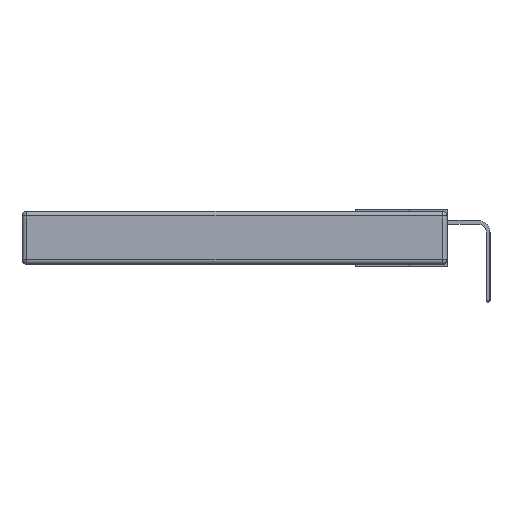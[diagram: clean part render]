
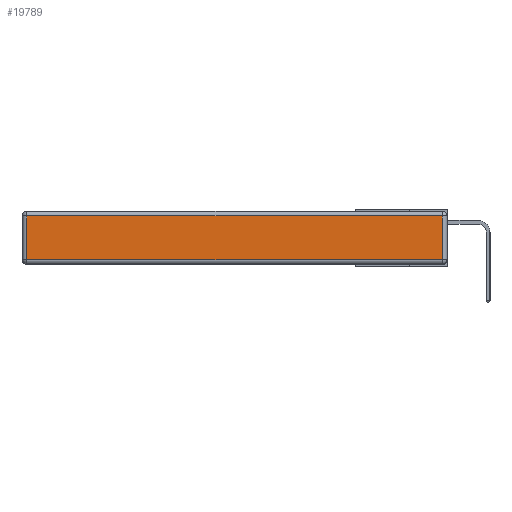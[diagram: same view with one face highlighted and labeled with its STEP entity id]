
A CAD part, left-side view. The second image highlights one B-rep face of the part: STEP entity #19789.
In plain terms, the highlighted planar face has unit normal (-1, 0, 0).
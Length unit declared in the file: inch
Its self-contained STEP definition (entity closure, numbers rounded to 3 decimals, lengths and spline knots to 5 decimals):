
#1203 = EDGE_CURVE ( 'NONE', #19280, #5224, #28338, .T. ) ;
#1354 = ORIENTED_EDGE ( 'NONE', *, *, #30653, .T. ) ;
#1513 = CARTESIAN_POINT ( 'NONE',  ( 0., 2.72, -0.343 ) ) ;
#2247 = CARTESIAN_POINT ( 'NONE',  ( 0., 2.72, -0.03 ) ) ;
#2945 = EDGE_CURVE ( 'NONE', #28315, #19280, #23787, .T. ) ;
#4897 = CARTESIAN_POINT ( 'NONE',  ( 0., 0., -0.343 ) ) ;
#5224 = VERTEX_POINT ( 'NONE', #20576 ) ;
#5275 = VECTOR ( 'NONE', #21024, 39.37008 ) ;
#6289 = EDGE_CURVE ( 'NONE', #5224, #21996, #17674, .T. ) ;
#6889 = LINE ( 'NONE', #13466, #11385 ) ;
#7324 = VECTOR ( 'NONE', #28319, 39.37008 ) ;
#9633 = AXIS2_PLACEMENT_3D ( 'NONE', #4897, #23283, #20837 ) ;
#9774 = FACE_OUTER_BOUND ( 'NONE', #18706, .T. ) ;
#11385 = VECTOR ( 'NONE', #18555, 39.37008 ) ;
#13466 = CARTESIAN_POINT ( 'NONE',  ( 0., 0.03, -0.343 ) ) ;
#15221 = ORIENTED_EDGE ( 'NONE', *, *, #6289, .T. ) ;
#17674 = LINE ( 'NONE', #26409, #22249 ) ;
#18404 = CARTESIAN_POINT ( 'NONE',  ( 0., 0.03, -0.03 ) ) ;
#18555 = DIRECTION ( 'NONE',  ( 0., 0., 1. ) ) ;
#18706 = EDGE_LOOP ( 'NONE', ( #15221, #1354, #28291, #32742 ) ) ;
#19280 = VERTEX_POINT ( 'NONE', #2247 ) ;
#19789 = ADVANCED_FACE ( 'NONE', ( #9774 ), #26167, .T. ) ;
#20576 = CARTESIAN_POINT ( 'NONE',  ( 0., 2.72, -0.313 ) ) ;
#20836 = DIRECTION ( 'NONE',  ( 0., -1., 0. ) ) ;
#20837 = DIRECTION ( 'NONE',  ( 0., 0., 1. ) ) ;
#21024 = DIRECTION ( 'NONE',  ( 0., 1., 0. ) ) ;
#21996 = VERTEX_POINT ( 'NONE', #33057 ) ;
#22249 = VECTOR ( 'NONE', #20836, 39.37008 ) ;
#23283 = DIRECTION ( 'NONE',  ( -1., 0., 0. ) ) ;
#23787 = LINE ( 'NONE', #32413, #5275 ) ;
#26167 = PLANE ( 'NONE',  #9633 ) ;
#26409 = CARTESIAN_POINT ( 'NONE',  ( 0., 0., -0.313 ) ) ;
#28291 = ORIENTED_EDGE ( 'NONE', *, *, #2945, .T. ) ;
#28315 = VERTEX_POINT ( 'NONE', #18404 ) ;
#28319 = DIRECTION ( 'NONE',  ( 0., 0., -1. ) ) ;
#28338 = LINE ( 'NONE', #1513, #7324 ) ;
#30653 = EDGE_CURVE ( 'NONE', #21996, #28315, #6889, .T. ) ;
#32413 = CARTESIAN_POINT ( 'NONE',  ( 0., 2.75, -0.03 ) ) ;
#32742 = ORIENTED_EDGE ( 'NONE', *, *, #1203, .T. ) ;
#33057 = CARTESIAN_POINT ( 'NONE',  ( 0., 0.03, -0.313 ) ) ;
